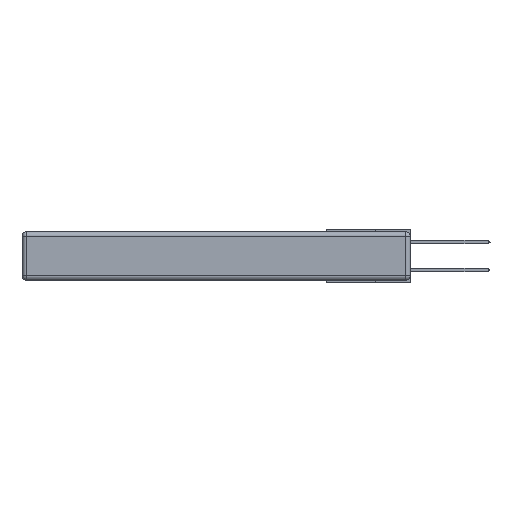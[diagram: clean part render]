
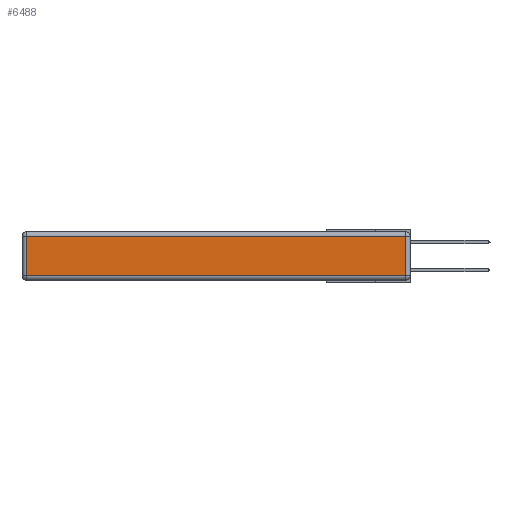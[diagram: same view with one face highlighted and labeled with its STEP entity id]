
A CAD part, left-side view. The second image highlights one B-rep face of the part: STEP entity #6488.
In plain terms, the highlighted planar face has unit normal (-1, 0, 0).
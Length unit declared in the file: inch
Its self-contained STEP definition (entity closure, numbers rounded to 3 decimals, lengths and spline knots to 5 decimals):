
#28 = CARTESIAN_POINT ( 'NONE',  ( 0., 0., -0.343 ) ) ;
#92 = ORIENTED_EDGE ( 'NONE', *, *, #849, .T. ) ;
#551 = CARTESIAN_POINT ( 'NONE',  ( 0., 0.03, -0.313 ) ) ;
#696 = FACE_OUTER_BOUND ( 'NONE', #4980, .T. ) ;
#849 = EDGE_CURVE ( 'NONE', #10946, #2307, #9613, .T. ) ;
#1453 = VECTOR ( 'NONE', #15656, 39.37008 ) ;
#2009 = CARTESIAN_POINT ( 'NONE',  ( 0., 0.03, -0.03 ) ) ;
#2077 = CARTESIAN_POINT ( 'NONE',  ( 0., 0., -0.313 ) ) ;
#2307 = VERTEX_POINT ( 'NONE', #13904 ) ;
#2330 = EDGE_CURVE ( 'NONE', #2307, #16101, #4189, .T. ) ;
#3077 = LINE ( 'NONE', #2077, #7094 ) ;
#3581 = CARTESIAN_POINT ( 'NONE',  ( 0., 2.72, -0.343 ) ) ;
#3585 = DIRECTION ( 'NONE',  ( 0., 0., 1. ) ) ;
#4189 = LINE ( 'NONE', #3581, #1453 ) ;
#4302 = ORIENTED_EDGE ( 'NONE', *, *, #19480, .T. ) ;
#4358 = CARTESIAN_POINT ( 'NONE',  ( 0., 2.72, -0.313 ) ) ;
#4980 = EDGE_LOOP ( 'NONE', ( #20311, #4302, #92, #11019 ) ) ;
#5033 = DIRECTION ( 'NONE',  ( 0., 1., 0. ) ) ;
#5455 = DIRECTION ( 'NONE',  ( -1., 0., 0. ) ) ;
#6488 = ADVANCED_FACE ( 'NONE', ( #696 ), #10365, .T. ) ;
#7094 = VECTOR ( 'NONE', #21099, 39.37008 ) ;
#9613 = LINE ( 'NONE', #10166, #14208 ) ;
#10166 = CARTESIAN_POINT ( 'NONE',  ( 0., 2.75, -0.03 ) ) ;
#10365 = PLANE ( 'NONE',  #21824 ) ;
#10914 = VECTOR ( 'NONE', #3585, 39.37008 ) ;
#10946 = VERTEX_POINT ( 'NONE', #2009 ) ;
#11019 = ORIENTED_EDGE ( 'NONE', *, *, #2330, .T. ) ;
#12117 = DIRECTION ( 'NONE',  ( 0., 0., 1. ) ) ;
#12642 = VERTEX_POINT ( 'NONE', #551 ) ;
#13904 = CARTESIAN_POINT ( 'NONE',  ( 0., 2.72, -0.03 ) ) ;
#13907 = CARTESIAN_POINT ( 'NONE',  ( 0., 0.03, -0.343 ) ) ;
#14208 = VECTOR ( 'NONE', #5033, 39.37008 ) ;
#15656 = DIRECTION ( 'NONE',  ( 0., 0., -1. ) ) ;
#16101 = VERTEX_POINT ( 'NONE', #4358 ) ;
#19480 = EDGE_CURVE ( 'NONE', #12642, #10946, #19600, .T. ) ;
#19600 = LINE ( 'NONE', #13907, #10914 ) ;
#19648 = EDGE_CURVE ( 'NONE', #16101, #12642, #3077, .T. ) ;
#20311 = ORIENTED_EDGE ( 'NONE', *, *, #19648, .T. ) ;
#21099 = DIRECTION ( 'NONE',  ( 0., -1., 0. ) ) ;
#21824 = AXIS2_PLACEMENT_3D ( 'NONE', #28, #5455, #12117 ) ;
